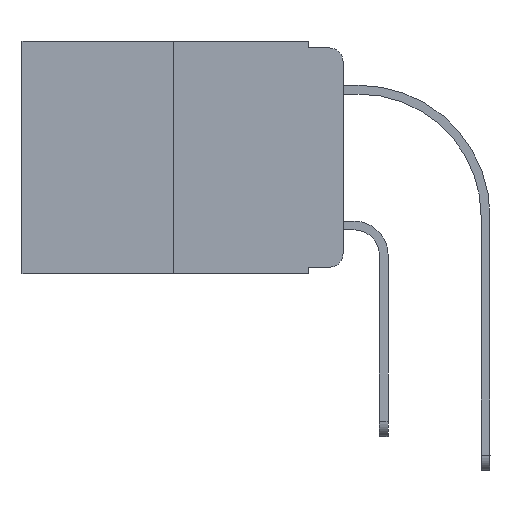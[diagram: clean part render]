
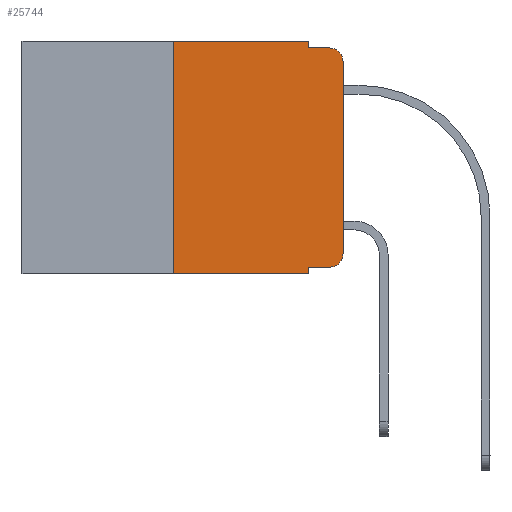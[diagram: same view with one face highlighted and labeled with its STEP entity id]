
A CAD part, left-side view. The second image highlights one B-rep face of the part: STEP entity #25744.
In plain terms, the highlighted planar face has unit normal (-1, 0, 0).
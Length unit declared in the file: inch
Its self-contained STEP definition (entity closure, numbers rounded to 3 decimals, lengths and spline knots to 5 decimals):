
#166 = VECTOR ( 'NONE', #401, 39.37008 ) ;
#401 = DIRECTION ( 'NONE',  ( 0., -1., 0. ) ) ;
#506 = ORIENTED_EDGE ( 'NONE', *, *, #5746, .F. ) ;
#696 = EDGE_CURVE ( 'NONE', #11979, #19878, #22110, .T. ) ;
#959 = PLANE ( 'NONE',  #8818 ) ;
#1041 = ORIENTED_EDGE ( 'NONE', *, *, #1850, .F. ) ;
#1507 = DIRECTION ( 'NONE',  ( 0., -1., 0. ) ) ;
#1780 = EDGE_CURVE ( 'NONE', #2722, #13322, #13218, .T. ) ;
#1850 = EDGE_CURVE ( 'NONE', #16165, #19878, #3012, .T. ) ;
#2433 = VERTEX_POINT ( 'NONE', #20188 ) ;
#2722 = VERTEX_POINT ( 'NONE', #3434 ) ;
#2771 = VECTOR ( 'NONE', #19233, 39.37008 ) ;
#3012 = LINE ( 'NONE', #21961, #8066 ) ;
#3239 = CARTESIAN_POINT ( 'NONE',  ( 0., 0.473, 0. ) ) ;
#3434 = CARTESIAN_POINT ( 'NONE',  ( 0., 0.25, 0. ) ) ;
#3503 = DIRECTION ( 'NONE',  ( 0., 0., 1. ) ) ;
#3619 = VECTOR ( 'NONE', #17997, 39.37008 ) ;
#3634 = CARTESIAN_POINT ( 'NONE',  ( 0., 0.25, 0. ) ) ;
#3718 = CARTESIAN_POINT ( 'NONE',  ( 0., 0., 0. ) ) ;
#3975 = DIRECTION ( 'NONE',  ( 0., 0., 1. ) ) ;
#4292 = CARTESIAN_POINT ( 'NONE',  ( 0., 0.473, -0.343 ) ) ;
#5607 = LINE ( 'NONE', #20012, #3619 ) ;
#5735 = VECTOR ( 'NONE', #3975, 39.37008 ) ;
#5746 = EDGE_CURVE ( 'NONE', #13322, #16165, #16799, .T. ) ;
#5931 = LINE ( 'NONE', #3634, #22996 ) ;
#6311 = CARTESIAN_POINT ( 'NONE',  ( 0., 0., -0.313 ) ) ;
#6856 = CARTESIAN_POINT ( 'NONE',  ( 0., 0.051, 0. ) ) ;
#7083 = CARTESIAN_POINT ( 'NONE',  ( 0., 0.051, -0.343 ) ) ;
#7219 = ORIENTED_EDGE ( 'NONE', *, *, #20462, .T. ) ;
#7329 = EDGE_CURVE ( 'NONE', #22519, #2722, #5931, .T. ) ;
#8038 = ORIENTED_EDGE ( 'NONE', *, *, #11904, .T. ) ;
#8051 = EDGE_CURVE ( 'NONE', #2433, #11755, #11736, .T. ) ;
#8066 = VECTOR ( 'NONE', #1507, 39.37008 ) ;
#8182 = DIRECTION ( 'NONE',  ( 0., 0., -1. ) ) ;
#8818 = AXIS2_PLACEMENT_3D ( 'NONE', #3239, #17129, #19668 ) ;
#10002 = CARTESIAN_POINT ( 'NONE',  ( 0., 0.25, -0.343 ) ) ;
#10065 = ORIENTED_EDGE ( 'NONE', *, *, #20053, .T. ) ;
#11466 = CARTESIAN_POINT ( 'NONE',  ( 0., 0.473, 0. ) ) ;
#11736 = LINE ( 'NONE', #19555, #13156 ) ;
#11755 = VERTEX_POINT ( 'NONE', #7083 ) ;
#11807 = AXIS2_PLACEMENT_3D ( 'NONE', #12602, #24089, #8182 ) ;
#11904 = EDGE_CURVE ( 'NONE', #12463, #11979, #24146, .T. ) ;
#11979 = VERTEX_POINT ( 'NONE', #23210 ) ;
#12015 = CARTESIAN_POINT ( 'NONE',  ( 0., 0.051, 0. ) ) ;
#12074 = ORIENTED_EDGE ( 'NONE', *, *, #8051, .F. ) ;
#12355 = ORIENTED_EDGE ( 'NONE', *, *, #20299, .T. ) ;
#12463 = VERTEX_POINT ( 'NONE', #6311 ) ;
#12602 = CARTESIAN_POINT ( 'NONE',  ( 0., 0.02, -0.03 ) ) ;
#12618 = CIRCLE ( 'NONE', #25055, 0.02 ) ;
#12787 = VECTOR ( 'NONE', #25716, 39.37008 ) ;
#12941 = VERTEX_POINT ( 'NONE', #26162 ) ;
#13156 = VECTOR ( 'NONE', #15505, 39.37008 ) ;
#13190 = ORIENTED_EDGE ( 'NONE', *, *, #696, .T. ) ;
#13218 = LINE ( 'NONE', #11466, #12787 ) ;
#13282 = DIRECTION ( 'NONE',  ( 0., 0., -1. ) ) ;
#13322 = VERTEX_POINT ( 'NONE', #12015 ) ;
#15505 = DIRECTION ( 'NONE',  ( 0., 0., -1. ) ) ;
#16165 = VERTEX_POINT ( 'NONE', #21291 ) ;
#16516 = CARTESIAN_POINT ( 'NONE',  ( 0., 0.02, -0.01 ) ) ;
#16799 = LINE ( 'NONE', #6856, #2771 ) ;
#17129 = DIRECTION ( 'NONE',  ( 1., 0., 0. ) ) ;
#17588 = CARTESIAN_POINT ( 'NONE',  ( 0., 0.02, -0.313 ) ) ;
#17997 = DIRECTION ( 'NONE',  ( 0., -1., 0. ) ) ;
#18273 = ORIENTED_EDGE ( 'NONE', *, *, #7329, .F. ) ;
#18657 = EDGE_LOOP ( 'NONE', ( #8038, #13190, #1041, #506, #23508, #18273, #10065, #12074, #7219, #12355 ) ) ;
#19073 = LINE ( 'NONE', #4292, #166 ) ;
#19233 = DIRECTION ( 'NONE',  ( 0., 0., -1. ) ) ;
#19555 = CARTESIAN_POINT ( 'NONE',  ( 0., 0.051, 0. ) ) ;
#19668 = DIRECTION ( 'NONE',  ( 0., 0., -1. ) ) ;
#19878 = VERTEX_POINT ( 'NONE', #16516 ) ;
#20012 = CARTESIAN_POINT ( 'NONE',  ( 0., 0.051, -0.333 ) ) ;
#20053 = EDGE_CURVE ( 'NONE', #22519, #11755, #19073, .T. ) ;
#20188 = CARTESIAN_POINT ( 'NONE',  ( 0., 0.051, -0.333 ) ) ;
#20299 = EDGE_CURVE ( 'NONE', #12941, #12463, #12618, .T. ) ;
#20462 = EDGE_CURVE ( 'NONE', #2433, #12941, #5607, .T. ) ;
#21291 = CARTESIAN_POINT ( 'NONE',  ( 0., 0.051, -0.01 ) ) ;
#21666 = FACE_OUTER_BOUND ( 'NONE', #18657, .T. ) ;
#21961 = CARTESIAN_POINT ( 'NONE',  ( 0., 0.051, -0.01 ) ) ;
#22110 = CIRCLE ( 'NONE', #11807, 0.02 ) ;
#22519 = VERTEX_POINT ( 'NONE', #10002 ) ;
#22996 = VECTOR ( 'NONE', #3503, 39.37008 ) ;
#23210 = CARTESIAN_POINT ( 'NONE',  ( 0., 0., -0.03 ) ) ;
#23508 = ORIENTED_EDGE ( 'NONE', *, *, #1780, .F. ) ;
#24089 = DIRECTION ( 'NONE',  ( -1., 0., 0. ) ) ;
#24146 = LINE ( 'NONE', #3718, #5735 ) ;
#25055 = AXIS2_PLACEMENT_3D ( 'NONE', #17588, #25778, #13282 ) ;
#25716 = DIRECTION ( 'NONE',  ( 0., -1., 0. ) ) ;
#25744 = ADVANCED_FACE ( 'NONE', ( #21666 ), #959, .F. ) ;
#25778 = DIRECTION ( 'NONE',  ( -1., 0., 0. ) ) ;
#26162 = CARTESIAN_POINT ( 'NONE',  ( 0., 0.02, -0.333 ) ) ;
